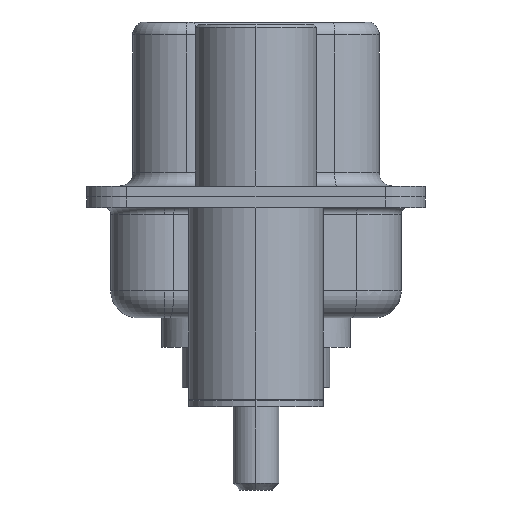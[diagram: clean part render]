
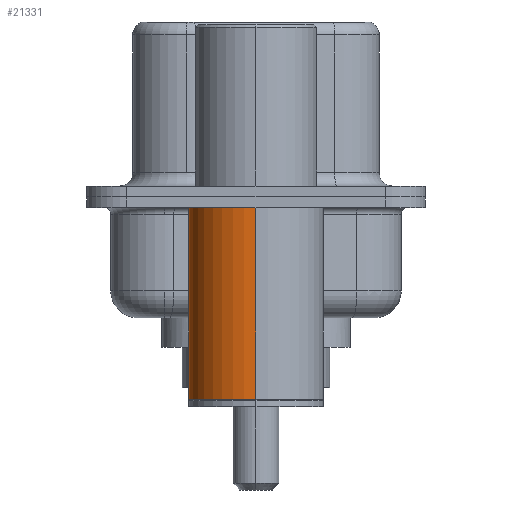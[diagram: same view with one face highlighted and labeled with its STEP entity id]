
A CAD part, left-side view. The second image highlights one B-rep face of the part: STEP entity #21331.
In plain terms, the highlighted cylindrical face has radius 2.5 mm (diameter 5 mm), a partial arc.
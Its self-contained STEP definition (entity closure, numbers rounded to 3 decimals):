
#831 = CARTESIAN_POINT ( 'NONE',  ( 0., 0., -0.4 ) ) ;
#877 = CARTESIAN_POINT ( 'NONE',  ( -2.5, 0., 0.581 ) ) ;
#1039 = CIRCLE ( 'NONE', #9810, 2.5 ) ;
#1265 = ORIENTED_EDGE ( 'NONE', *, *, #15711, .T. ) ;
#2514 = DIRECTION ( 'NONE',  ( 1., 0., 0. ) ) ;
#2566 = DIRECTION ( 'NONE',  ( 0., 0., 1. ) ) ;
#2986 = AXIS2_PLACEMENT_3D ( 'NONE', #4685, #16163, #6388 ) ;
#3021 = VERTEX_POINT ( 'NONE', #6315 ) ;
#3515 = DIRECTION ( 'NONE',  ( 0., 0., 1. ) ) ;
#3705 = CARTESIAN_POINT ( 'NONE',  ( -2.5, 0., -0.4 ) ) ;
#3973 = CARTESIAN_POINT ( 'NONE',  ( -2.5, 0., -7.525 ) ) ;
#4424 = ORIENTED_EDGE ( 'NONE', *, *, #11781, .F. ) ;
#4548 = CARTESIAN_POINT ( 'NONE',  ( 2.5, 0., -0.4 ) ) ;
#4685 = CARTESIAN_POINT ( 'NONE',  ( 0., 0., -7.525 ) ) ;
#5499 = EDGE_LOOP ( 'NONE', ( #17880, #1265, #4424, #16473 ) ) ;
#6315 = CARTESIAN_POINT ( 'NONE',  ( 2.5, 0., -7.525 ) ) ;
#6388 = DIRECTION ( 'NONE',  ( 1., 0., 0. ) ) ;
#8781 = FACE_OUTER_BOUND ( 'NONE', #5499, .T. ) ;
#9810 = AXIS2_PLACEMENT_3D ( 'NONE', #831, #12451, #2514 ) ;
#10605 = VECTOR ( 'NONE', #12392, 1000. ) ;
#10715 = CARTESIAN_POINT ( 'NONE',  ( 2.5, 0., 0.581 ) ) ;
#11705 = VERTEX_POINT ( 'NONE', #3973 ) ;
#11781 = EDGE_CURVE ( 'NONE', #16987, #15028, #1039, .T. ) ;
#12392 = DIRECTION ( 'NONE',  ( 0., 0., 1. ) ) ;
#12451 = DIRECTION ( 'NONE',  ( 0., 0., 1. ) ) ;
#12504 = EDGE_CURVE ( 'NONE', #3021, #11705, #21213, .T. ) ;
#13433 = CARTESIAN_POINT ( 'NONE',  ( 0., 0., 0.581 ) ) ;
#15028 = VERTEX_POINT ( 'NONE', #3705 ) ;
#15053 = DIRECTION ( 'NONE',  ( 1., 0., 0. ) ) ;
#15711 = EDGE_CURVE ( 'NONE', #11705, #15028, #15757, .T. ) ;
#15757 = LINE ( 'NONE', #877, #20616 ) ;
#16163 = DIRECTION ( 'NONE',  ( 0., 0., 1. ) ) ;
#16406 = CYLINDRICAL_SURFACE ( 'NONE', #21037, 2.5 ) ;
#16473 = ORIENTED_EDGE ( 'NONE', *, *, #17450, .F. ) ;
#16987 = VERTEX_POINT ( 'NONE', #4548 ) ;
#17450 = EDGE_CURVE ( 'NONE', #3021, #16987, #19296, .T. ) ;
#17880 = ORIENTED_EDGE ( 'NONE', *, *, #12504, .T. ) ;
#19296 = LINE ( 'NONE', #10715, #10605 ) ;
#20616 = VECTOR ( 'NONE', #2566, 1000. ) ;
#21037 = AXIS2_PLACEMENT_3D ( 'NONE', #13433, #3515, #15053 ) ;
#21213 = CIRCLE ( 'NONE', #2986, 2.5 ) ;
#21331 = ADVANCED_FACE ( 'NONE', ( #8781 ), #16406, .T. ) ;
